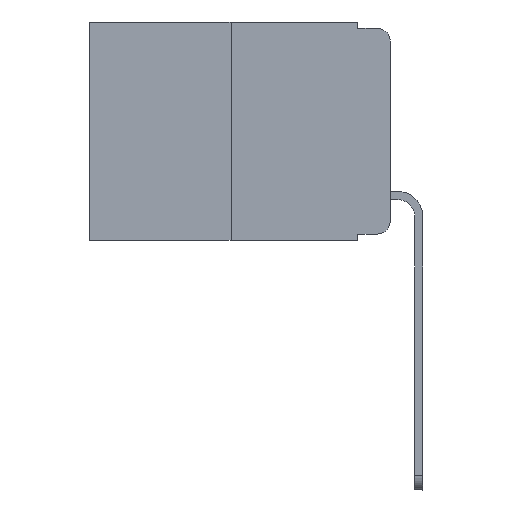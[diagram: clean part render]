
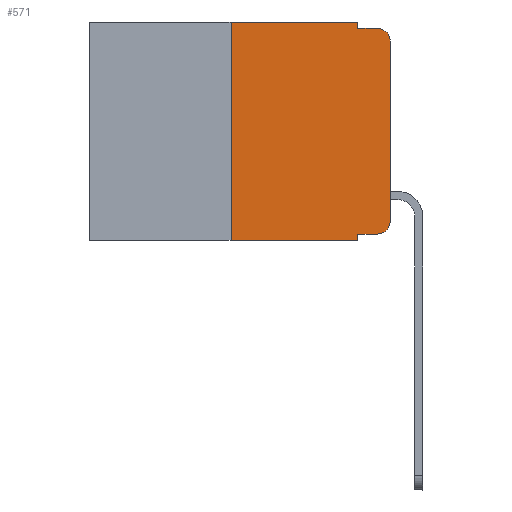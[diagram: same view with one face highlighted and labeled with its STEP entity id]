
A CAD part, left-side view. The second image highlights one B-rep face of the part: STEP entity #571.
In plain terms, the highlighted planar face has unit normal (-1, 0, 0).
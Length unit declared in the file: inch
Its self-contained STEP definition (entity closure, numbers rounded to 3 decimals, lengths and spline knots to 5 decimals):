
#169 = CARTESIAN_POINT ( 'NONE',  ( 0., 0.473, 0. ) ) ;
#270 = ORIENTED_EDGE ( 'NONE', *, *, #8458, .F. ) ;
#376 = LINE ( 'NONE', #169, #4791 ) ;
#414 = LINE ( 'NONE', #4371, #5536 ) ;
#451 = EDGE_CURVE ( 'NONE', #8048, #9063, #376, .T. ) ;
#571 = ADVANCED_FACE ( 'NONE', ( #1440 ), #7877, .F. ) ;
#799 = CIRCLE ( 'NONE', #8547, 0.02 ) ;
#903 = VERTEX_POINT ( 'NONE', #2752 ) ;
#1130 = VERTEX_POINT ( 'NONE', #5771 ) ;
#1327 = VECTOR ( 'NONE', #5018, 39.37008 ) ;
#1348 = VECTOR ( 'NONE', #2136, 39.37008 ) ;
#1440 = FACE_OUTER_BOUND ( 'NONE', #2112, .T. ) ;
#1458 = ORIENTED_EDGE ( 'NONE', *, *, #8134, .T. ) ;
#1537 = DIRECTION ( 'NONE',  ( 0., 0., -1. ) ) ;
#1828 = CARTESIAN_POINT ( 'NONE',  ( 0., 0.25, 0. ) ) ;
#1913 = VECTOR ( 'NONE', #3163, 39.37008 ) ;
#1998 = ORIENTED_EDGE ( 'NONE', *, *, #7075, .T. ) ;
#2112 = EDGE_LOOP ( 'NONE', ( #7036, #9605, #270, #7841, #10070, #10021, #1458, #10408, #3292, #1998 ) ) ;
#2124 = EDGE_CURVE ( 'NONE', #9063, #7918, #6344, .T. ) ;
#2136 = DIRECTION ( 'NONE',  ( 0., -1., 0. ) ) ;
#2276 = VERTEX_POINT ( 'NONE', #8612 ) ;
#2280 = DIRECTION ( 'NONE',  ( 0., 0., 1. ) ) ;
#2345 = CARTESIAN_POINT ( 'NONE',  ( 0., 0.02, -0.03 ) ) ;
#2356 = DIRECTION ( 'NONE',  ( 0., 0., -1. ) ) ;
#2425 = LINE ( 'NONE', #3111, #7812 ) ;
#2491 = EDGE_CURVE ( 'NONE', #3531, #2276, #799, .T. ) ;
#2752 = CARTESIAN_POINT ( 'NONE',  ( 0., 0.25, -0.343 ) ) ;
#2950 = CARTESIAN_POINT ( 'NONE',  ( 0., 0.25, 0. ) ) ;
#2985 = DIRECTION ( 'NONE',  ( 1., 0., 0. ) ) ;
#3034 = LINE ( 'NONE', #7082, #1348 ) ;
#3069 = DIRECTION ( 'NONE',  ( -1., 0., 0. ) ) ;
#3099 = VERTEX_POINT ( 'NONE', #3858 ) ;
#3111 = CARTESIAN_POINT ( 'NONE',  ( 0., 0.051, -0.333 ) ) ;
#3163 = DIRECTION ( 'NONE',  ( 0., -1., 0. ) ) ;
#3292 = ORIENTED_EDGE ( 'NONE', *, *, #8170, .T. ) ;
#3531 = VERTEX_POINT ( 'NONE', #7871 ) ;
#3614 = CARTESIAN_POINT ( 'NONE',  ( 0., 0.051, 0. ) ) ;
#3823 = CARTESIAN_POINT ( 'NONE',  ( 0., 0.02, -0.313 ) ) ;
#3858 = CARTESIAN_POINT ( 'NONE',  ( 0., 0.051, -0.333 ) ) ;
#3893 = EDGE_CURVE ( 'NONE', #3099, #4980, #414, .T. ) ;
#3973 = VECTOR ( 'NONE', #2356, 39.37008 ) ;
#4371 = CARTESIAN_POINT ( 'NONE',  ( 0., 0.051, 0. ) ) ;
#4376 = CIRCLE ( 'NONE', #6570, 0.02 ) ;
#4387 = DIRECTION ( 'NONE',  ( 0., -1., 0. ) ) ;
#4791 = VECTOR ( 'NONE', #4387, 39.37008 ) ;
#4810 = CARTESIAN_POINT ( 'NONE',  ( 0., 0.051, 0. ) ) ;
#4980 = VERTEX_POINT ( 'NONE', #9078 ) ;
#5013 = CARTESIAN_POINT ( 'NONE',  ( 0., 0.02, -0.333 ) ) ;
#5018 = DIRECTION ( 'NONE',  ( 0., 0., 1. ) ) ;
#5070 = LINE ( 'NONE', #1828, #1327 ) ;
#5145 = DIRECTION ( 'NONE',  ( 0., 0., -1. ) ) ;
#5331 = DIRECTION ( 'NONE',  ( 0., 0., -1. ) ) ;
#5536 = VECTOR ( 'NONE', #5145, 39.37008 ) ;
#5771 = CARTESIAN_POINT ( 'NONE',  ( 0., 0., -0.313 ) ) ;
#6009 = EDGE_CURVE ( 'NONE', #903, #8048, #5070, .T. ) ;
#6344 = LINE ( 'NONE', #4810, #3973 ) ;
#6385 = DIRECTION ( 'NONE',  ( 0., 0., -1. ) ) ;
#6570 = AXIS2_PLACEMENT_3D ( 'NONE', #3823, #3069, #1537 ) ;
#6807 = CARTESIAN_POINT ( 'NONE',  ( 0., 0.473, 0. ) ) ;
#7036 = ORIENTED_EDGE ( 'NONE', *, *, #7080, .T. ) ;
#7058 = LINE ( 'NONE', #9515, #9954 ) ;
#7075 = EDGE_CURVE ( 'NONE', #8258, #1130, #4376, .T. ) ;
#7080 = EDGE_CURVE ( 'NONE', #1130, #3531, #7058, .T. ) ;
#7082 = CARTESIAN_POINT ( 'NONE',  ( 0., 0.051, -0.01 ) ) ;
#7812 = VECTOR ( 'NONE', #8801, 39.37008 ) ;
#7841 = ORIENTED_EDGE ( 'NONE', *, *, #2124, .F. ) ;
#7871 = CARTESIAN_POINT ( 'NONE',  ( 0., 0., -0.03 ) ) ;
#7877 = PLANE ( 'NONE',  #10200 ) ;
#7918 = VERTEX_POINT ( 'NONE', #10015 ) ;
#7958 = CARTESIAN_POINT ( 'NONE',  ( 0., 0.473, -0.343 ) ) ;
#7977 = DIRECTION ( 'NONE',  ( -1., 0., 0. ) ) ;
#8048 = VERTEX_POINT ( 'NONE', #2950 ) ;
#8134 = EDGE_CURVE ( 'NONE', #903, #4980, #9457, .T. ) ;
#8170 = EDGE_CURVE ( 'NONE', #3099, #8258, #2425, .T. ) ;
#8258 = VERTEX_POINT ( 'NONE', #5013 ) ;
#8458 = EDGE_CURVE ( 'NONE', #7918, #2276, #3034, .T. ) ;
#8547 = AXIS2_PLACEMENT_3D ( 'NONE', #2345, #7977, #6385 ) ;
#8612 = CARTESIAN_POINT ( 'NONE',  ( 0., 0.02, -0.01 ) ) ;
#8801 = DIRECTION ( 'NONE',  ( 0., -1., 0. ) ) ;
#9063 = VERTEX_POINT ( 'NONE', #3614 ) ;
#9078 = CARTESIAN_POINT ( 'NONE',  ( 0., 0.051, -0.343 ) ) ;
#9457 = LINE ( 'NONE', #7958, #1913 ) ;
#9515 = CARTESIAN_POINT ( 'NONE',  ( 0., 0., 0. ) ) ;
#9605 = ORIENTED_EDGE ( 'NONE', *, *, #2491, .T. ) ;
#9954 = VECTOR ( 'NONE', #2280, 39.37008 ) ;
#10015 = CARTESIAN_POINT ( 'NONE',  ( 0., 0.051, -0.01 ) ) ;
#10021 = ORIENTED_EDGE ( 'NONE', *, *, #6009, .F. ) ;
#10070 = ORIENTED_EDGE ( 'NONE', *, *, #451, .F. ) ;
#10200 = AXIS2_PLACEMENT_3D ( 'NONE', #6807, #2985, #5331 ) ;
#10408 = ORIENTED_EDGE ( 'NONE', *, *, #3893, .F. ) ;
